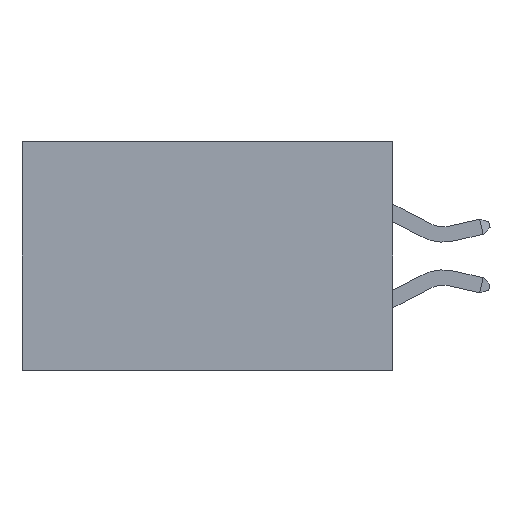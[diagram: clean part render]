
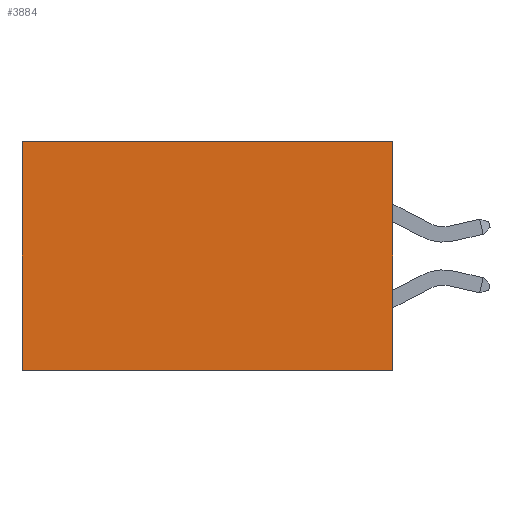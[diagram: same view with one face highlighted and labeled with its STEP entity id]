
A CAD part, left-side view. The second image highlights one B-rep face of the part: STEP entity #3884.
In plain terms, the highlighted planar face has unit normal (-1, 0, 0).
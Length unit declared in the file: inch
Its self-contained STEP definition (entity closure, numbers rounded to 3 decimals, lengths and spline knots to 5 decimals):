
#539 = AXIS2_PLACEMENT_3D ( 'NONE', #10895, #3620, #3073 ) ;
#574 = DIRECTION ( 'NONE',  ( 0., 0., -1. ) ) ;
#2124 = VERTEX_POINT ( 'NONE', #8507 ) ;
#2272 = VECTOR ( 'NONE', #12795, 39.37008 ) ;
#3073 = DIRECTION ( 'NONE',  ( 0., 0., -1. ) ) ;
#3141 = LINE ( 'NONE', #13989, #8874 ) ;
#3258 = LINE ( 'NONE', #6504, #8652 ) ;
#3264 = CARTESIAN_POINT ( 'NONE',  ( 0.2875, 0., 0. ) ) ;
#3294 = LINE ( 'NONE', #9670, #13970 ) ;
#3620 = DIRECTION ( 'NONE',  ( 1., 0., 0. ) ) ;
#3884 = ADVANCED_FACE ( 'NONE', ( #12563 ), #5528, .F. ) ;
#4346 = EDGE_CURVE ( 'NONE', #11887, #13714, #3141, .T. ) ;
#4367 = CARTESIAN_POINT ( 'NONE',  ( 0.2875, 0.6, 0. ) ) ;
#5199 = VERTEX_POINT ( 'NONE', #13259 ) ;
#5528 = PLANE ( 'NONE',  #539 ) ;
#5606 = ORIENTED_EDGE ( 'NONE', *, *, #7661, .T. ) ;
#6359 = ORIENTED_EDGE ( 'NONE', *, *, #9170, .F. ) ;
#6504 = CARTESIAN_POINT ( 'NONE',  ( 0.2875, 0., 0. ) ) ;
#7661 = EDGE_CURVE ( 'NONE', #13714, #5199, #3294, .T. ) ;
#8507 = CARTESIAN_POINT ( 'NONE',  ( 0.2875, 0., -0.37 ) ) ;
#8652 = VECTOR ( 'NONE', #574, 39.37008 ) ;
#8720 = CARTESIAN_POINT ( 'NONE',  ( 0.2875, 0., -0.37 ) ) ;
#8874 = VECTOR ( 'NONE', #13903, 39.37008 ) ;
#9170 = EDGE_CURVE ( 'NONE', #11887, #2124, #3258, .T. ) ;
#9218 = ORIENTED_EDGE ( 'NONE', *, *, #4346, .T. ) ;
#9670 = CARTESIAN_POINT ( 'NONE',  ( 0.2875, 0.6, 0. ) ) ;
#9789 = EDGE_LOOP ( 'NONE', ( #5606, #11667, #6359, #9218 ) ) ;
#10445 = EDGE_CURVE ( 'NONE', #2124, #5199, #11223, .T. ) ;
#10715 = DIRECTION ( 'NONE',  ( 0., 0., -1. ) ) ;
#10895 = CARTESIAN_POINT ( 'NONE',  ( 0.2875, 0., 0. ) ) ;
#11223 = LINE ( 'NONE', #8720, #2272 ) ;
#11667 = ORIENTED_EDGE ( 'NONE', *, *, #10445, .F. ) ;
#11887 = VERTEX_POINT ( 'NONE', #3264 ) ;
#12563 = FACE_OUTER_BOUND ( 'NONE', #9789, .T. ) ;
#12795 = DIRECTION ( 'NONE',  ( 0., 1., 0. ) ) ;
#13259 = CARTESIAN_POINT ( 'NONE',  ( 0.2875, 0.6, -0.37 ) ) ;
#13714 = VERTEX_POINT ( 'NONE', #4367 ) ;
#13903 = DIRECTION ( 'NONE',  ( 0., 1., 0. ) ) ;
#13970 = VECTOR ( 'NONE', #10715, 39.37008 ) ;
#13989 = CARTESIAN_POINT ( 'NONE',  ( 0.2875, 0., 0. ) ) ;
